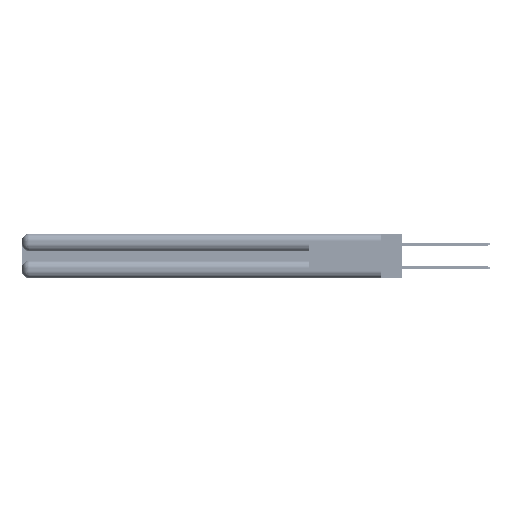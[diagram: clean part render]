
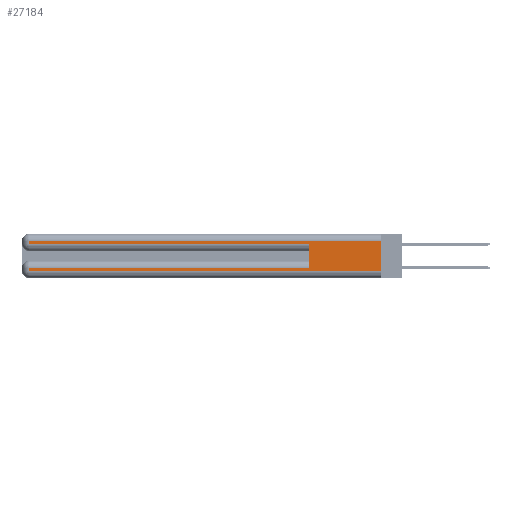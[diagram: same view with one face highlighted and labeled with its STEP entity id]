
A CAD part, left-side view. The second image highlights one B-rep face of the part: STEP entity #27184.
In plain terms, the highlighted planar face has unit normal (-1, 0, 0).
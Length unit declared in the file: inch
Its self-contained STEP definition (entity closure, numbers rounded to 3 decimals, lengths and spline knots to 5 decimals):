
#1461 = FACE_OUTER_BOUND ( 'NONE', #37533, .T. ) ;
#2340 = EDGE_CURVE ( 'NONE', #11956, #5917, #18422, .T. ) ;
#2520 = CARTESIAN_POINT ( 'NONE',  ( 0., 0.6, 0.285 ) ) ;
#2907 = CARTESIAN_POINT ( 'NONE',  ( 0., 0.6, 0.145 ) ) ;
#3358 = DIRECTION ( 'NONE',  ( 0., 1., 0. ) ) ;
#5413 = CARTESIAN_POINT ( 'NONE',  ( 0., 2.94, 0.37 ) ) ;
#5535 = VERTEX_POINT ( 'NONE', #50698 ) ;
#5784 = PLANE ( 'NONE',  #33607 ) ;
#5917 = VERTEX_POINT ( 'NONE', #44781 ) ;
#7372 = VECTOR ( 'NONE', #17938, 39.37008 ) ;
#7754 = LINE ( 'NONE', #12213, #28441 ) ;
#7983 = EDGE_CURVE ( 'NONE', #5535, #31871, #18843, .T. ) ;
#8741 = EDGE_CURVE ( 'NONE', #35019, #17778, #14148, .T. ) ;
#11577 = VECTOR ( 'NONE', #33719, 39.37008 ) ;
#11681 = CARTESIAN_POINT ( 'NONE',  ( 0., 0., 0.31 ) ) ;
#11956 = VERTEX_POINT ( 'NONE', #51501 ) ;
#12213 = CARTESIAN_POINT ( 'NONE',  ( 0., 2.94, 0.37 ) ) ;
#12828 = VECTOR ( 'NONE', #47835, 39.37008 ) ;
#14085 = CARTESIAN_POINT ( 'NONE',  ( 0., 0., 0.37 ) ) ;
#14148 = LINE ( 'NONE', #23364, #12828 ) ;
#14660 = DIRECTION ( 'NONE',  ( 0., 0., -1. ) ) ;
#14885 = ORIENTED_EDGE ( 'NONE', *, *, #40791, .F. ) ;
#15019 = CARTESIAN_POINT ( 'NONE',  ( 0., 0., 0.37 ) ) ;
#15838 = EDGE_CURVE ( 'NONE', #5917, #31364, #39292, .T. ) ;
#16394 = DIRECTION ( 'NONE',  ( 0., 0., -1. ) ) ;
#16782 = DIRECTION ( 'NONE',  ( 0., -1., 0. ) ) ;
#17288 = ORIENTED_EDGE ( 'NONE', *, *, #26700, .F. ) ;
#17778 = VERTEX_POINT ( 'NONE', #51568 ) ;
#17938 = DIRECTION ( 'NONE',  ( 0., 0., -1. ) ) ;
#18305 = DIRECTION ( 'NONE',  ( 0., 0., -1. ) ) ;
#18422 = LINE ( 'NONE', #5413, #7372 ) ;
#18517 = ORIENTED_EDGE ( 'NONE', *, *, #15838, .T. ) ;
#18843 = LINE ( 'NONE', #28339, #48901 ) ;
#20182 = ORIENTED_EDGE ( 'NONE', *, *, #39564, .T. ) ;
#21014 = ORIENTED_EDGE ( 'NONE', *, *, #34121, .T. ) ;
#23364 = CARTESIAN_POINT ( 'NONE',  ( 0., 0., 0.085 ) ) ;
#23614 = DIRECTION ( 'NONE',  ( 0., 0., 1. ) ) ;
#24575 = VERTEX_POINT ( 'NONE', #39736 ) ;
#24731 = VECTOR ( 'NONE', #14660, 39.37008 ) ;
#26019 = CARTESIAN_POINT ( 'NONE',  ( 0., 0., 0.06 ) ) ;
#26700 = EDGE_CURVE ( 'NONE', #35019, #31364, #34440, .T. ) ;
#27184 = ADVANCED_FACE ( 'NONE', ( #1461 ), #5784, .F. ) ;
#28339 = CARTESIAN_POINT ( 'NONE',  ( 0., 0., 0.06 ) ) ;
#28441 = VECTOR ( 'NONE', #16394, 39.37008 ) ;
#29332 = LINE ( 'NONE', #11681, #51071 ) ;
#29619 = CARTESIAN_POINT ( 'NONE',  ( 0., 0., 0.285 ) ) ;
#30814 = ORIENTED_EDGE ( 'NONE', *, *, #2340, .T. ) ;
#31075 = ORIENTED_EDGE ( 'NONE', *, *, #7983, .T. ) ;
#31364 = VERTEX_POINT ( 'NONE', #2520 ) ;
#31871 = VERTEX_POINT ( 'NONE', #26019 ) ;
#33607 = AXIS2_PLACEMENT_3D ( 'NONE', #14085, #42855, #18305 ) ;
#33719 = DIRECTION ( 'NONE',  ( 0., -1., 0. ) ) ;
#34121 = EDGE_CURVE ( 'NONE', #17778, #5535, #7754, .T. ) ;
#34440 = LINE ( 'NONE', #2907, #45302 ) ;
#35019 = VERTEX_POINT ( 'NONE', #37924 ) ;
#37533 = EDGE_LOOP ( 'NONE', ( #14885, #20182, #30814, #18517, #17288, #50525, #21014, #31075 ) ) ;
#37924 = CARTESIAN_POINT ( 'NONE',  ( 0., 0.6, 0.085 ) ) ;
#39292 = LINE ( 'NONE', #29619, #11577 ) ;
#39564 = EDGE_CURVE ( 'NONE', #24575, #11956, #29332, .T. ) ;
#39736 = CARTESIAN_POINT ( 'NONE',  ( 0., 0., 0.31 ) ) ;
#40791 = EDGE_CURVE ( 'NONE', #24575, #31871, #46482, .T. ) ;
#42855 = DIRECTION ( 'NONE',  ( 1., 0., 0. ) ) ;
#44781 = CARTESIAN_POINT ( 'NONE',  ( 0., 2.94, 0.285 ) ) ;
#45302 = VECTOR ( 'NONE', #23614, 39.37008 ) ;
#46482 = LINE ( 'NONE', #15019, #24731 ) ;
#47835 = DIRECTION ( 'NONE',  ( 0., 1., 0. ) ) ;
#48901 = VECTOR ( 'NONE', #16782, 39.37008 ) ;
#50525 = ORIENTED_EDGE ( 'NONE', *, *, #8741, .T. ) ;
#50698 = CARTESIAN_POINT ( 'NONE',  ( 0., 2.94, 0.06 ) ) ;
#51071 = VECTOR ( 'NONE', #3358, 39.37008 ) ;
#51501 = CARTESIAN_POINT ( 'NONE',  ( 0., 2.94, 0.31 ) ) ;
#51568 = CARTESIAN_POINT ( 'NONE',  ( 0., 2.94, 0.085 ) ) ;
